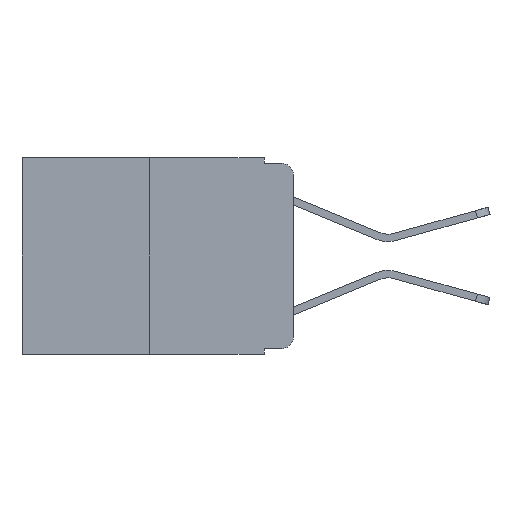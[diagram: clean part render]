
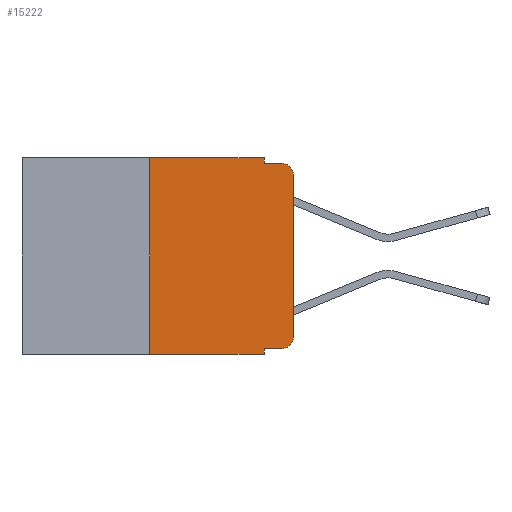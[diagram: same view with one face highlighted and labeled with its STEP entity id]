
A CAD part, left-side view. The second image highlights one B-rep face of the part: STEP entity #15222.
In plain terms, the highlighted planar face has unit normal (-1, 0, 0).
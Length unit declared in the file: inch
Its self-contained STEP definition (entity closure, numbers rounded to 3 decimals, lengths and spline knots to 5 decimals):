
#165 = ORIENTED_EDGE ( 'NONE', *, *, #1266, .F. ) ;
#256 = VECTOR ( 'NONE', #17094, 39.37008 ) ;
#264 = EDGE_CURVE ( 'NONE', #4077, #5533, #11850, .T. ) ;
#1075 = VECTOR ( 'NONE', #6727, 39.37008 ) ;
#1266 = EDGE_CURVE ( 'NONE', #4077, #12199, #15433, .T. ) ;
#2009 = AXIS2_PLACEMENT_3D ( 'NONE', #14127, #6348, #15391 ) ;
#2078 = CARTESIAN_POINT ( 'NONE',  ( 0., 0.051, 0. ) ) ;
#2249 = EDGE_CURVE ( 'NONE', #8528, #10781, #16664, .T. ) ;
#2282 = VECTOR ( 'NONE', #3384, 39.37008 ) ;
#2696 = CARTESIAN_POINT ( 'NONE',  ( 0., 0.051, -0.333 ) ) ;
#2771 = VERTEX_POINT ( 'NONE', #15986 ) ;
#3156 = EDGE_CURVE ( 'NONE', #7614, #3591, #14203, .T. ) ;
#3209 = CARTESIAN_POINT ( 'NONE',  ( 0., 0.051, 0. ) ) ;
#3316 = DIRECTION ( 'NONE',  ( 0., 0., -1. ) ) ;
#3384 = DIRECTION ( 'NONE',  ( 0., -1., 0. ) ) ;
#3591 = VERTEX_POINT ( 'NONE', #9037 ) ;
#3674 = CARTESIAN_POINT ( 'NONE',  ( 0., 0.051, 0. ) ) ;
#3953 = CARTESIAN_POINT ( 'NONE',  ( 0., 0.473, 0. ) ) ;
#4077 = VERTEX_POINT ( 'NONE', #2696 ) ;
#4106 = EDGE_CURVE ( 'NONE', #3591, #15615, #11216, .T. ) ;
#4339 = CARTESIAN_POINT ( 'NONE',  ( 0., 0., -0.313 ) ) ;
#4704 = VERTEX_POINT ( 'NONE', #4339 ) ;
#5010 = ORIENTED_EDGE ( 'NONE', *, *, #16564, .T. ) ;
#5038 = EDGE_CURVE ( 'NONE', #2771, #15615, #16952, .T. ) ;
#5044 = DIRECTION ( 'NONE',  ( 0., 0., -1. ) ) ;
#5054 = VECTOR ( 'NONE', #3316, 39.37008 ) ;
#5393 = ORIENTED_EDGE ( 'NONE', *, *, #2249, .F. ) ;
#5438 = CARTESIAN_POINT ( 'NONE',  ( 0., 0.25, 0. ) ) ;
#5533 = VERTEX_POINT ( 'NONE', #9973 ) ;
#5937 = EDGE_CURVE ( 'NONE', #4704, #2771, #11122, .T. ) ;
#6341 = DIRECTION ( 'NONE',  ( -1., 0., 0. ) ) ;
#6348 = DIRECTION ( 'NONE',  ( -1., 0., 0. ) ) ;
#6414 = FACE_OUTER_BOUND ( 'NONE', #12902, .T. ) ;
#6727 = DIRECTION ( 'NONE',  ( 0., 0., 1. ) ) ;
#6806 = LINE ( 'NONE', #7522, #2282 ) ;
#6933 = CARTESIAN_POINT ( 'NONE',  ( 0., 0.051, -0.333 ) ) ;
#7522 = CARTESIAN_POINT ( 'NONE',  ( 0., 0.473, 0. ) ) ;
#7614 = VERTEX_POINT ( 'NONE', #3674 ) ;
#8403 = EDGE_CURVE ( 'NONE', #8528, #12199, #16654, .T. ) ;
#8457 = CARTESIAN_POINT ( 'NONE',  ( 0., 0.25, -0.343 ) ) ;
#8490 = VECTOR ( 'NONE', #16487, 39.37008 ) ;
#8528 = VERTEX_POINT ( 'NONE', #8457 ) ;
#9037 = CARTESIAN_POINT ( 'NONE',  ( 0., 0.051, -0.01 ) ) ;
#9198 = ORIENTED_EDGE ( 'NONE', *, *, #8403, .T. ) ;
#9259 = ORIENTED_EDGE ( 'NONE', *, *, #16478, .F. ) ;
#9301 = ORIENTED_EDGE ( 'NONE', *, *, #264, .T. ) ;
#9440 = DIRECTION ( 'NONE',  ( 0., 0., -1. ) ) ;
#9539 = CIRCLE ( 'NONE', #2009, 0.02 ) ;
#9973 = CARTESIAN_POINT ( 'NONE',  ( 0., 0.02, -0.333 ) ) ;
#10781 = VERTEX_POINT ( 'NONE', #5438 ) ;
#11122 = LINE ( 'NONE', #14482, #1075 ) ;
#11216 = LINE ( 'NONE', #16942, #256 ) ;
#11850 = LINE ( 'NONE', #6933, #8490 ) ;
#12199 = VERTEX_POINT ( 'NONE', #15903 ) ;
#12600 = ORIENTED_EDGE ( 'NONE', *, *, #5937, .T. ) ;
#12769 = ORIENTED_EDGE ( 'NONE', *, *, #4106, .F. ) ;
#12902 = EDGE_LOOP ( 'NONE', ( #12600, #16824, #12769, #12970, #9259, #5393, #9198, #165, #9301, #5010 ) ) ;
#12970 = ORIENTED_EDGE ( 'NONE', *, *, #3156, .F. ) ;
#13389 = VECTOR ( 'NONE', #17008, 39.37008 ) ;
#13392 = VECTOR ( 'NONE', #14611, 39.37008 ) ;
#13792 = VECTOR ( 'NONE', #5044, 39.37008 ) ;
#14124 = CARTESIAN_POINT ( 'NONE',  ( 0., 0.02, -0.03 ) ) ;
#14127 = CARTESIAN_POINT ( 'NONE',  ( 0., 0.02, -0.313 ) ) ;
#14203 = LINE ( 'NONE', #2078, #13792 ) ;
#14482 = CARTESIAN_POINT ( 'NONE',  ( 0., 0., 0. ) ) ;
#14574 = CARTESIAN_POINT ( 'NONE',  ( 0., 0.25, 0. ) ) ;
#14609 = CARTESIAN_POINT ( 'NONE',  ( 0., 0.473, -0.343 ) ) ;
#14611 = DIRECTION ( 'NONE',  ( 0., 0., 1. ) ) ;
#15141 = CARTESIAN_POINT ( 'NONE',  ( 0., 0.02, -0.01 ) ) ;
#15174 = AXIS2_PLACEMENT_3D ( 'NONE', #3953, #16896, #9440 ) ;
#15222 = ADVANCED_FACE ( 'NONE', ( #6414 ), #15694, .F. ) ;
#15388 = DIRECTION ( 'NONE',  ( 0., 0., -1. ) ) ;
#15391 = DIRECTION ( 'NONE',  ( 0., 0., -1. ) ) ;
#15433 = LINE ( 'NONE', #3209, #5054 ) ;
#15615 = VERTEX_POINT ( 'NONE', #15141 ) ;
#15694 = PLANE ( 'NONE',  #15174 ) ;
#15903 = CARTESIAN_POINT ( 'NONE',  ( 0., 0.051, -0.343 ) ) ;
#15986 = CARTESIAN_POINT ( 'NONE',  ( 0., 0., -0.03 ) ) ;
#16341 = AXIS2_PLACEMENT_3D ( 'NONE', #14124, #6341, #15388 ) ;
#16478 = EDGE_CURVE ( 'NONE', #10781, #7614, #6806, .T. ) ;
#16487 = DIRECTION ( 'NONE',  ( 0., -1., 0. ) ) ;
#16564 = EDGE_CURVE ( 'NONE', #5533, #4704, #9539, .T. ) ;
#16654 = LINE ( 'NONE', #14609, #13389 ) ;
#16664 = LINE ( 'NONE', #14574, #13392 ) ;
#16824 = ORIENTED_EDGE ( 'NONE', *, *, #5038, .T. ) ;
#16896 = DIRECTION ( 'NONE',  ( 1., 0., 0. ) ) ;
#16942 = CARTESIAN_POINT ( 'NONE',  ( 0., 0.051, -0.01 ) ) ;
#16952 = CIRCLE ( 'NONE', #16341, 0.02 ) ;
#17008 = DIRECTION ( 'NONE',  ( 0., -1., 0. ) ) ;
#17094 = DIRECTION ( 'NONE',  ( 0., -1., 0. ) ) ;
